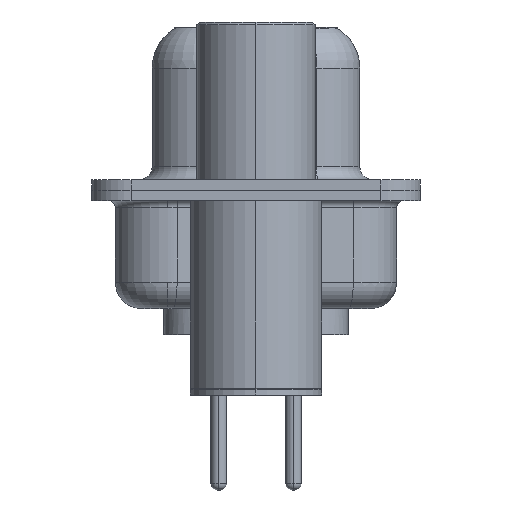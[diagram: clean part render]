
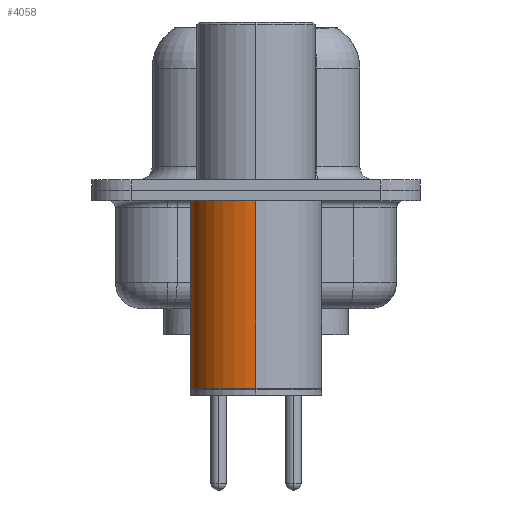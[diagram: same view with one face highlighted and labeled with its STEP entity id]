
A CAD part, left-side view. The second image highlights one B-rep face of the part: STEP entity #4058.
In plain terms, the highlighted cylindrical face has radius 2.5 mm (diameter 5 mm), a partial arc.
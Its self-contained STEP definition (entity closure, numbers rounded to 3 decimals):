
#355 = CARTESIAN_POINT ( 'NONE',  ( 2.5, 0., -7.525 ) ) ;
#370 = CIRCLE ( 'NONE', #14151, 2.5 ) ;
#497 = ORIENTED_EDGE ( 'NONE', *, *, #3188, .F. ) ;
#938 = DIRECTION ( 'NONE',  ( 0., 0., 1. ) ) ;
#1198 = VERTEX_POINT ( 'NONE', #15412 ) ;
#1644 = DIRECTION ( 'NONE',  ( 0., 0., 1. ) ) ;
#3188 = EDGE_CURVE ( 'NONE', #13764, #24022, #370, .T. ) ;
#3232 = AXIS2_PLACEMENT_3D ( 'NONE', #12296, #938, #27728 ) ;
#4058 = ADVANCED_FACE ( 'NONE', ( #5684 ), #27169, .T. ) ;
#4835 = LINE ( 'NONE', #9305, #12587 ) ;
#5251 = CARTESIAN_POINT ( 'NONE',  ( -2.5, 0., -0.4 ) ) ;
#5557 = ORIENTED_EDGE ( 'NONE', *, *, #5797, .T. ) ;
#5684 = FACE_OUTER_BOUND ( 'NONE', #12615, .T. ) ;
#5797 = EDGE_CURVE ( 'NONE', #24604, #1198, #6301, .T. ) ;
#6301 = CIRCLE ( 'NONE', #12254, 2.5 ) ;
#6400 = CARTESIAN_POINT ( 'NONE',  ( 2.5, 0., 0.581 ) ) ;
#7909 = CARTESIAN_POINT ( 'NONE',  ( 0., 0., -7.525 ) ) ;
#8723 = EDGE_CURVE ( 'NONE', #1198, #24022, #4835, .T. ) ;
#9029 = EDGE_CURVE ( 'NONE', #24604, #13764, #17023, .T. ) ;
#9305 = CARTESIAN_POINT ( 'NONE',  ( -2.5, 0., 0.581 ) ) ;
#12221 = DIRECTION ( 'NONE',  ( 0., 0., 1. ) ) ;
#12254 = AXIS2_PLACEMENT_3D ( 'NONE', #7909, #25483, #16651 ) ;
#12296 = CARTESIAN_POINT ( 'NONE',  ( 0., 0., 0.581 ) ) ;
#12587 = VECTOR ( 'NONE', #18188, 1000. ) ;
#12615 = EDGE_LOOP ( 'NONE', ( #5557, #26805, #497, #14508 ) ) ;
#13764 = VERTEX_POINT ( 'NONE', #19768 ) ;
#14151 = AXIS2_PLACEMENT_3D ( 'NONE', #16368, #12221, #18545 ) ;
#14508 = ORIENTED_EDGE ( 'NONE', *, *, #9029, .F. ) ;
#15412 = CARTESIAN_POINT ( 'NONE',  ( -2.5, 0., -7.525 ) ) ;
#16368 = CARTESIAN_POINT ( 'NONE',  ( 0., 0., -0.4 ) ) ;
#16651 = DIRECTION ( 'NONE',  ( 1., 0., 0. ) ) ;
#17023 = LINE ( 'NONE', #6400, #23193 ) ;
#18188 = DIRECTION ( 'NONE',  ( 0., 0., 1. ) ) ;
#18545 = DIRECTION ( 'NONE',  ( 1., 0., 0. ) ) ;
#19768 = CARTESIAN_POINT ( 'NONE',  ( 2.5, 0., -0.4 ) ) ;
#23193 = VECTOR ( 'NONE', #1644, 1000. ) ;
#24022 = VERTEX_POINT ( 'NONE', #5251 ) ;
#24604 = VERTEX_POINT ( 'NONE', #355 ) ;
#25483 = DIRECTION ( 'NONE',  ( 0., 0., 1. ) ) ;
#26805 = ORIENTED_EDGE ( 'NONE', *, *, #8723, .T. ) ;
#27169 = CYLINDRICAL_SURFACE ( 'NONE', #3232, 2.5 ) ;
#27728 = DIRECTION ( 'NONE',  ( 1., 0., 0. ) ) ;
